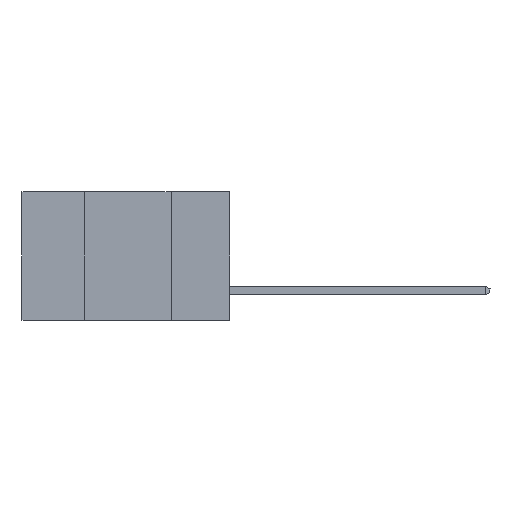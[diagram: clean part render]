
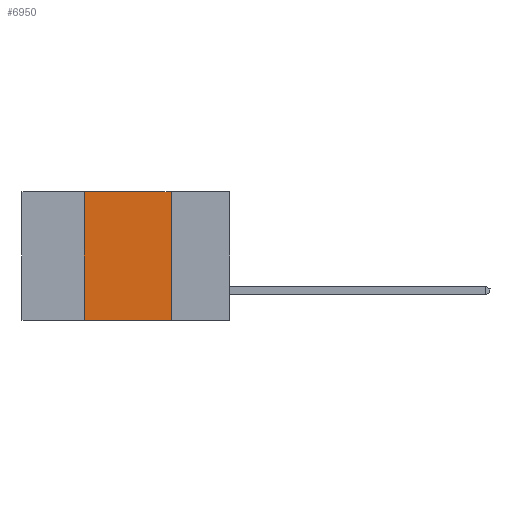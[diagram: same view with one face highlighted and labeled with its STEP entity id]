
A CAD part, left-side view. The second image highlights one B-rep face of the part: STEP entity #6950.
In plain terms, the highlighted planar face has unit normal (-1, 0, 0).
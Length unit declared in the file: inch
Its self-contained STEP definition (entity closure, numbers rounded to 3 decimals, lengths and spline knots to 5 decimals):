
#144 = FACE_OUTER_BOUND ( 'NONE', #4334, .T. ) ;
#403 = CARTESIAN_POINT ( 'NONE',  ( 0., 0.6, 0. ) ) ;
#1392 = ORIENTED_EDGE ( 'NONE', *, *, #4062, .F. ) ;
#1691 = EDGE_CURVE ( 'NONE', #6788, #7159, #7304, .T. ) ;
#1851 = LINE ( 'NONE', #3850, #5852 ) ;
#2355 = EDGE_CURVE ( 'NONE', #8473, #4900, #2532, .T. ) ;
#2472 = ORIENTED_EDGE ( 'NONE', *, *, #2355, .F. ) ;
#2532 = LINE ( 'NONE', #7321, #4344 ) ;
#2552 = VECTOR ( 'NONE', #4065, 39.37008 ) ;
#2780 = CARTESIAN_POINT ( 'NONE',  ( 0., 0.6, 0. ) ) ;
#3043 = DIRECTION ( 'NONE',  ( 0., -1., 0. ) ) ;
#3210 = EDGE_CURVE ( 'NONE', #6788, #4900, #1851, .T. ) ;
#3681 = CARTESIAN_POINT ( 'NONE',  ( 0., 0.17, -0.37 ) ) ;
#3764 = DIRECTION ( 'NONE',  ( 0., -1., 0. ) ) ;
#3850 = CARTESIAN_POINT ( 'NONE',  ( 0., 0.6, -0.37 ) ) ;
#3980 = CARTESIAN_POINT ( 'NONE',  ( 0., 0.42, -0.37 ) ) ;
#4062 = EDGE_CURVE ( 'NONE', #7159, #8473, #4974, .T. ) ;
#4065 = DIRECTION ( 'NONE',  ( 0., 0., 1. ) ) ;
#4334 = EDGE_LOOP ( 'NONE', ( #2472, #1392, #8168, #6800 ) ) ;
#4344 = VECTOR ( 'NONE', #6024, 39.37008 ) ;
#4900 = VERTEX_POINT ( 'NONE', #3681 ) ;
#4974 = LINE ( 'NONE', #403, #7900 ) ;
#5401 = DIRECTION ( 'NONE',  ( 1., 0., 0. ) ) ;
#5804 = AXIS2_PLACEMENT_3D ( 'NONE', #2780, #5401, #7261 ) ;
#5849 = CARTESIAN_POINT ( 'NONE',  ( 0., 0.17, 0. ) ) ;
#5852 = VECTOR ( 'NONE', #3764, 39.37008 ) ;
#6024 = DIRECTION ( 'NONE',  ( 0., 0., -1. ) ) ;
#6788 = VERTEX_POINT ( 'NONE', #7742 ) ;
#6800 = ORIENTED_EDGE ( 'NONE', *, *, #3210, .T. ) ;
#6950 = ADVANCED_FACE ( 'NONE', ( #144 ), #8094, .F. ) ;
#7159 = VERTEX_POINT ( 'NONE', #8438 ) ;
#7261 = DIRECTION ( 'NONE',  ( 0., 0., -1. ) ) ;
#7304 = LINE ( 'NONE', #3980, #2552 ) ;
#7321 = CARTESIAN_POINT ( 'NONE',  ( 0., 0.17, -0.37 ) ) ;
#7742 = CARTESIAN_POINT ( 'NONE',  ( 0., 0.42, -0.37 ) ) ;
#7900 = VECTOR ( 'NONE', #3043, 39.37008 ) ;
#8094 = PLANE ( 'NONE',  #5804 ) ;
#8168 = ORIENTED_EDGE ( 'NONE', *, *, #1691, .F. ) ;
#8438 = CARTESIAN_POINT ( 'NONE',  ( 0., 0.42, 0. ) ) ;
#8473 = VERTEX_POINT ( 'NONE', #5849 ) ;
